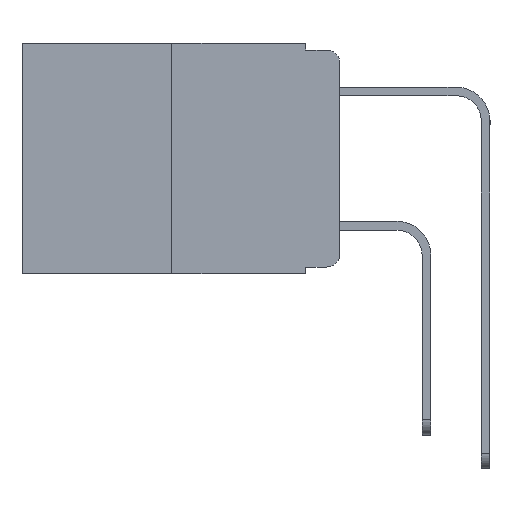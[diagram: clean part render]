
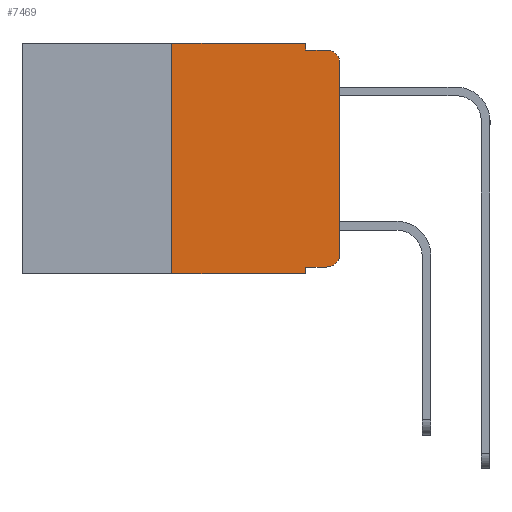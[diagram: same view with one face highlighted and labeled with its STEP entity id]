
A CAD part, left-side view. The second image highlights one B-rep face of the part: STEP entity #7469.
In plain terms, the highlighted planar face has unit normal (-1, 0, 0).
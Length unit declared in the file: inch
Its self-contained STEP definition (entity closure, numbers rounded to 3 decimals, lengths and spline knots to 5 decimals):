
#95 = EDGE_CURVE ( 'NONE', #5275, #7467, #1545, .T. ) ;
#563 = DIRECTION ( 'NONE',  ( 0., 0., 1. ) ) ;
#566 = CARTESIAN_POINT ( 'NONE',  ( 0., 0., 0. ) ) ;
#649 = EDGE_CURVE ( 'NONE', #2797, #9577, #1508, .T. ) ;
#699 = LINE ( 'NONE', #5979, #8965 ) ;
#730 = EDGE_LOOP ( 'NONE', ( #1124, #1183, #1257, #1347, #1398, #1457, #1653, #1782, #2029, #5506 ) ) ;
#736 = VECTOR ( 'NONE', #9325, 39.37008 ) ;
#801 = DIRECTION ( 'NONE',  ( 0., 0., -1. ) ) ;
#1091 = LINE ( 'NONE', #566, #11944 ) ;
#1124 = ORIENTED_EDGE ( 'NONE', *, *, #1509, .T. ) ;
#1183 = ORIENTED_EDGE ( 'NONE', *, *, #649, .T. ) ;
#1231 = DIRECTION ( 'NONE',  ( -1., 0., 0. ) ) ;
#1257 = ORIENTED_EDGE ( 'NONE', *, *, #13077, .F. ) ;
#1347 = ORIENTED_EDGE ( 'NONE', *, *, #12515, .F. ) ;
#1398 = ORIENTED_EDGE ( 'NONE', *, *, #95, .F. ) ;
#1457 = ORIENTED_EDGE ( 'NONE', *, *, #11936, .F. ) ;
#1508 = CIRCLE ( 'NONE', #10094, 0.02 ) ;
#1509 = EDGE_CURVE ( 'NONE', #2798, #2797, #1091, .T. ) ;
#1524 = CARTESIAN_POINT ( 'NONE',  ( 0., 0.25, 0. ) ) ;
#1545 = LINE ( 'NONE', #10602, #736 ) ;
#1653 = ORIENTED_EDGE ( 'NONE', *, *, #3914, .T. ) ;
#1782 = ORIENTED_EDGE ( 'NONE', *, *, #11353, .F. ) ;
#2029 = ORIENTED_EDGE ( 'NONE', *, *, #10752, .T. ) ;
#2405 = VERTEX_POINT ( 'NONE', #10203 ) ;
#2598 = CARTESIAN_POINT ( 'NONE',  ( 0., 0.051, -0.333 ) ) ;
#2605 = VERTEX_POINT ( 'NONE', #12492 ) ;
#2797 = VERTEX_POINT ( 'NONE', #4923 ) ;
#2798 = VERTEX_POINT ( 'NONE', #4877 ) ;
#3032 = DIRECTION ( 'NONE',  ( 0., 0., -1. ) ) ;
#3373 = LINE ( 'NONE', #7252, #3742 ) ;
#3742 = VECTOR ( 'NONE', #3032, 39.37008 ) ;
#3914 = EDGE_CURVE ( 'NONE', #12685, #2605, #699, .T. ) ;
#4450 = CARTESIAN_POINT ( 'NONE',  ( 0., 0.051, -0.01 ) ) ;
#4766 = CIRCLE ( 'NONE', #4908, 0.02 ) ;
#4877 = CARTESIAN_POINT ( 'NONE',  ( 0., 0., -0.313 ) ) ;
#4908 = AXIS2_PLACEMENT_3D ( 'NONE', #7775, #1231, #8729 ) ;
#4923 = CARTESIAN_POINT ( 'NONE',  ( 0., 0., -0.03 ) ) ;
#5091 = VECTOR ( 'NONE', #11028, 39.37008 ) ;
#5242 = CARTESIAN_POINT ( 'NONE',  ( 0., 0.051, -0.333 ) ) ;
#5275 = VERTEX_POINT ( 'NONE', #13189 ) ;
#5506 = ORIENTED_EDGE ( 'NONE', *, *, #10132, .T. ) ;
#5869 = VECTOR ( 'NONE', #7557, 39.37008 ) ;
#5979 = CARTESIAN_POINT ( 'NONE',  ( 0., 0.473, -0.343 ) ) ;
#6407 = CARTESIAN_POINT ( 'NONE',  ( 0., 0.051, 0. ) ) ;
#6737 = VERTEX_POINT ( 'NONE', #10019 ) ;
#7156 = CARTESIAN_POINT ( 'NONE',  ( 0., 0.02, -0.03 ) ) ;
#7252 = CARTESIAN_POINT ( 'NONE',  ( 0., 0.051, 0. ) ) ;
#7451 = DIRECTION ( 'NONE',  ( 1., 0., 0. ) ) ;
#7467 = VERTEX_POINT ( 'NONE', #6407 ) ;
#7469 = ADVANCED_FACE ( 'NONE', ( #10352 ), #12899, .F. ) ;
#7557 = DIRECTION ( 'NONE',  ( 0., -1., 0. ) ) ;
#7685 = DIRECTION ( 'NONE',  ( 0., 0., -1. ) ) ;
#7775 = CARTESIAN_POINT ( 'NONE',  ( 0., 0.02, -0.313 ) ) ;
#7868 = AXIS2_PLACEMENT_3D ( 'NONE', #12035, #7451, #801 ) ;
#8632 = CARTESIAN_POINT ( 'NONE',  ( 0., 0.051, 0. ) ) ;
#8729 = DIRECTION ( 'NONE',  ( 0., 0., -1. ) ) ;
#8965 = VECTOR ( 'NONE', #9231, 39.37008 ) ;
#8980 = VECTOR ( 'NONE', #10798, 39.37008 ) ;
#9231 = DIRECTION ( 'NONE',  ( 0., -1., 0. ) ) ;
#9325 = DIRECTION ( 'NONE',  ( 0., -1., 0. ) ) ;
#9577 = VERTEX_POINT ( 'NONE', #12615 ) ;
#10019 = CARTESIAN_POINT ( 'NONE',  ( 0., 0.02, -0.333 ) ) ;
#10094 = AXIS2_PLACEMENT_3D ( 'NONE', #7156, #10718, #10704 ) ;
#10132 = EDGE_CURVE ( 'NONE', #6737, #2798, #4766, .T. ) ;
#10203 = CARTESIAN_POINT ( 'NONE',  ( 0., 0.051, -0.01 ) ) ;
#10290 = LINE ( 'NONE', #5242, #5091 ) ;
#10352 = FACE_OUTER_BOUND ( 'NONE', #730, .T. ) ;
#10602 = CARTESIAN_POINT ( 'NONE',  ( 0., 0.473, 0. ) ) ;
#10665 = CARTESIAN_POINT ( 'NONE',  ( 0., 0.25, -0.343 ) ) ;
#10704 = DIRECTION ( 'NONE',  ( 0., 0., -1. ) ) ;
#10718 = DIRECTION ( 'NONE',  ( -1., 0., 0. ) ) ;
#10752 = EDGE_CURVE ( 'NONE', #11861, #6737, #10290, .T. ) ;
#10798 = DIRECTION ( 'NONE',  ( 0., 0., 1. ) ) ;
#11028 = DIRECTION ( 'NONE',  ( 0., -1., 0. ) ) ;
#11353 = EDGE_CURVE ( 'NONE', #11861, #2605, #3373, .T. ) ;
#11692 = LINE ( 'NONE', #1524, #8980 ) ;
#11861 = VERTEX_POINT ( 'NONE', #2598 ) ;
#11936 = EDGE_CURVE ( 'NONE', #12685, #5275, #11692, .T. ) ;
#11944 = VECTOR ( 'NONE', #563, 39.37008 ) ;
#11947 = VECTOR ( 'NONE', #7685, 39.37008 ) ;
#12035 = CARTESIAN_POINT ( 'NONE',  ( 0., 0.473, 0. ) ) ;
#12213 = LINE ( 'NONE', #8632, #11947 ) ;
#12492 = CARTESIAN_POINT ( 'NONE',  ( 0., 0.051, -0.343 ) ) ;
#12515 = EDGE_CURVE ( 'NONE', #7467, #2405, #12213, .T. ) ;
#12615 = CARTESIAN_POINT ( 'NONE',  ( 0., 0.02, -0.01 ) ) ;
#12685 = VERTEX_POINT ( 'NONE', #10665 ) ;
#12899 = PLANE ( 'NONE',  #7868 ) ;
#13008 = LINE ( 'NONE', #4450, #5869 ) ;
#13077 = EDGE_CURVE ( 'NONE', #2405, #9577, #13008, .T. ) ;
#13189 = CARTESIAN_POINT ( 'NONE',  ( 0., 0.25, 0. ) ) ;
